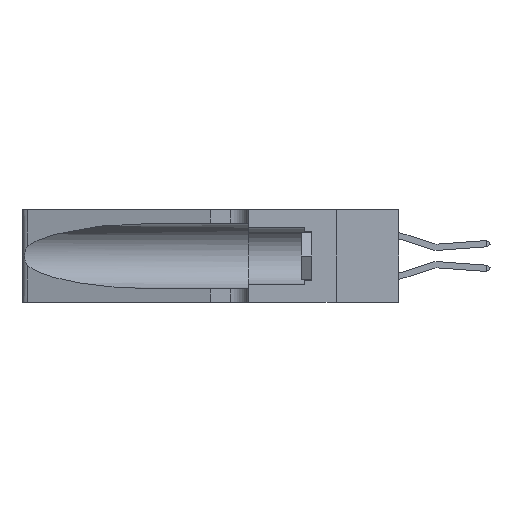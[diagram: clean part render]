
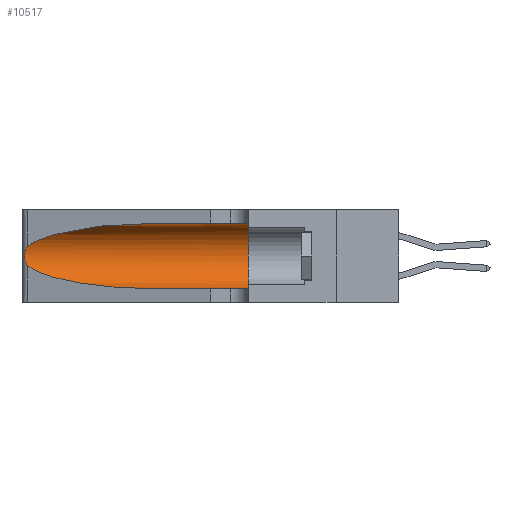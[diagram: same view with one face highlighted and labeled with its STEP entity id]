
A CAD part, left-side view. The second image highlights one B-rep face of the part: STEP entity #10517.
In plain terms, the highlighted cylindrical face has radius 3.308 mm (diameter 6.617 mm), a partial arc.
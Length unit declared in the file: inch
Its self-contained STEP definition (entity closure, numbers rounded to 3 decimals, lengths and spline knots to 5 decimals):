
#342 =( BOUNDED_CURVE ( )  B_SPLINE_CURVE ( 3, ( #559, #14095, #27897, #10256 ),
 .UNSPECIFIED., .F., .T. ) 
 B_SPLINE_CURVE_WITH_KNOTS ( ( 4, 4 ),
 ( 3.44316, 4.71239 ),
 .UNSPECIFIED. ) 
 CURVE ( )  GEOMETRIC_REPRESENTATION_ITEM ( )  RATIONAL_B_SPLINE_CURVE ( ( 1., 0.87, 0.87, 1. ) ) 
 REPRESENTATION_ITEM ( '' )  );
#559 = CARTESIAN_POINT ( 'NONE',  ( 0.25487, 1.22718, 0.14631 ) ) ;
#731 = CYLINDRICAL_SURFACE ( 'NONE', #2216, 0.13025 ) ;
#1449 =( BOUNDED_CURVE ( )  B_SPLINE_CURVE ( 3, ( #19832, #22501, #25131, #9156 ),
 .UNSPECIFIED., .F., .T. ) 
 B_SPLINE_CURVE_WITH_KNOTS ( ( 4, 4 ),
 ( 1.5708, 2.84003 ),
 .UNSPECIFIED. ) 
 CURVE ( )  GEOMETRIC_REPRESENTATION_ITEM ( )  RATIONAL_B_SPLINE_CURVE ( ( 1., 0.87, 0.87, 1. ) ) 
 REPRESENTATION_ITEM ( '' )  );
#1595 = DIRECTION ( 'NONE',  ( 0., 0., 1. ) ) ;
#1601 = FACE_OUTER_BOUND ( 'NONE', #4345, .T. ) ;
#1689 = EDGE_CURVE ( 'NONE', #8952, #18286, #342, .T. ) ;
#1985 = CARTESIAN_POINT ( 'NONE',  ( 0.26017, 1.23833, 0.17102 ) ) ;
#2048 = CARTESIAN_POINT ( 'NONE',  ( 0.1305, 0.72297, 0.31525 ) ) ;
#2216 = AXIS2_PLACEMENT_3D ( 'NONE', #30127, #14254, #8827 ) ;
#2761 = EDGE_CURVE ( 'NONE', #33352, #22773, #32976, .T. ) ;
#3137 = ORIENTED_EDGE ( 'NONE', *, *, #29196, .T. ) ;
#4345 = EDGE_LOOP ( 'NONE', ( #16651, #3137, #11198, #25383, #27033, #13718 ) ) ;
#4758 = CARTESIAN_POINT ( 'NONE',  ( 0.25789, 1.23486, 0.15765 ) ) ;
#5657 = VECTOR ( 'NONE', #19360, 39.37008 ) ;
#5799 = CARTESIAN_POINT ( 'NONE',  ( 0.1305, 1.61858, 0.31525 ) ) ;
#6446 = EDGE_CURVE ( 'NONE', #10162, #33352, #26591, .T. ) ;
#6543 = LINE ( 'NONE', #32476, #5657 ) ;
#6677 = CARTESIAN_POINT ( 'NONE',  ( 0.1305, 0.35, 0.05475 ) ) ;
#7495 = CARTESIAN_POINT ( 'NONE',  ( 0.25555, 1.22993, 0.14849 ) ) ;
#7801 = B_SPLINE_CURVE_WITH_KNOTS ( 'NONE', 3,
 ( #23412, #10077, #28714, #12760, #31333, #15485, #33938, #18200, #1985, #20864, #4758, #23508, #7495, #26157 ),
 .UNSPECIFIED., .F., .F.,
 ( 4, 2, 2, 2, 2, 2, 4 ),
 ( 0., 0.00027, 0.00053, 0.00107, 0.0016, 0.00187, 0.00214 ),
 .UNSPECIFIED. ) ;
#8508 = DIRECTION ( 'NONE',  ( 0., -1., 0. ) ) ;
#8827 = DIRECTION ( 'NONE',  ( 0., 0., -1. ) ) ;
#8952 = VERTEX_POINT ( 'NONE', #10320 ) ;
#9156 = CARTESIAN_POINT ( 'NONE',  ( 0.25487, 1.22718, 0.22369 ) ) ;
#10077 = CARTESIAN_POINT ( 'NONE',  ( 0.25555, 1.22994, 0.2215 ) ) ;
#10162 = VERTEX_POINT ( 'NONE', #2048 ) ;
#10256 = CARTESIAN_POINT ( 'NONE',  ( 0.1305, 0.72297, 0.05475 ) ) ;
#10320 = CARTESIAN_POINT ( 'NONE',  ( 0.25487, 1.22718, 0.14631 ) ) ;
#10517 = ADVANCED_FACE ( 'NONE', ( #1601 ), #731, .F. ) ;
#11198 = ORIENTED_EDGE ( 'NONE', *, *, #1689, .T. ) ;
#11284 = CARTESIAN_POINT ( 'NONE',  ( 0.1305, 0.72297, 0.05475 ) ) ;
#12760 = CARTESIAN_POINT ( 'NONE',  ( 0.25787, 1.23484, 0.2124 ) ) ;
#13718 = ORIENTED_EDGE ( 'NONE', *, *, #6446, .F. ) ;
#13776 = CARTESIAN_POINT ( 'NONE',  ( 0.1305, 0.35, 0.31525 ) ) ;
#14095 = CARTESIAN_POINT ( 'NONE',  ( 0.2373, 1.15595, 0.08982 ) ) ;
#14254 = DIRECTION ( 'NONE',  ( 0., -1., 0. ) ) ;
#15485 = CARTESIAN_POINT ( 'NONE',  ( 0.26018, 1.23835, 0.19895 ) ) ;
#16026 = VERTEX_POINT ( 'NONE', #32435 ) ;
#16651 = ORIENTED_EDGE ( 'NONE', *, *, #30262, .T. ) ;
#17809 = DIRECTION ( 'NONE',  ( 0., 1., 0. ) ) ;
#18200 = CARTESIAN_POINT ( 'NONE',  ( 0.26075, 1.23896, 0.178 ) ) ;
#18286 = VERTEX_POINT ( 'NONE', #11284 ) ;
#19360 = DIRECTION ( 'NONE',  ( 0., -1., 0. ) ) ;
#19583 = VECTOR ( 'NONE', #8508, 39.37008 ) ;
#19832 = CARTESIAN_POINT ( 'NONE',  ( 0.1305, 0.72297, 0.31525 ) ) ;
#20864 = CARTESIAN_POINT ( 'NONE',  ( 0.25856, 1.23593, 0.16098 ) ) ;
#22501 = CARTESIAN_POINT ( 'NONE',  ( 0.18966, 0.96281, 0.31525 ) ) ;
#22773 = VERTEX_POINT ( 'NONE', #6677 ) ;
#23412 = CARTESIAN_POINT ( 'NONE',  ( 0.25487, 1.22718, 0.22369 ) ) ;
#23508 = CARTESIAN_POINT ( 'NONE',  ( 0.25639, 1.23186, 0.15144 ) ) ;
#25131 = CARTESIAN_POINT ( 'NONE',  ( 0.2373, 1.15595, 0.28018 ) ) ;
#25383 = ORIENTED_EDGE ( 'NONE', *, *, #32046, .T. ) ;
#26157 = CARTESIAN_POINT ( 'NONE',  ( 0.25487, 1.22718, 0.14631 ) ) ;
#26591 = LINE ( 'NONE', #5799, #19583 ) ;
#27033 = ORIENTED_EDGE ( 'NONE', *, *, #2761, .F. ) ;
#27897 = CARTESIAN_POINT ( 'NONE',  ( 0.18966, 0.96281, 0.05475 ) ) ;
#28714 = CARTESIAN_POINT ( 'NONE',  ( 0.25639, 1.23184, 0.21858 ) ) ;
#29196 = EDGE_CURVE ( 'NONE', #16026, #8952, #7801, .T. ) ;
#30127 = CARTESIAN_POINT ( 'NONE',  ( 0.1305, 1.61858, 0.185 ) ) ;
#30262 = EDGE_CURVE ( 'NONE', #10162, #16026, #1449, .T. ) ;
#31333 = CARTESIAN_POINT ( 'NONE',  ( 0.25854, 1.2359, 0.20912 ) ) ;
#32046 = EDGE_CURVE ( 'NONE', #18286, #22773, #6543, .T. ) ;
#32435 = CARTESIAN_POINT ( 'NONE',  ( 0.25487, 1.22718, 0.22369 ) ) ;
#32476 = CARTESIAN_POINT ( 'NONE',  ( 0.1305, 1.61858, 0.05475 ) ) ;
#32976 = CIRCLE ( 'NONE', #33580, 0.13025 ) ;
#33352 = VERTEX_POINT ( 'NONE', #13776 ) ;
#33568 = CARTESIAN_POINT ( 'NONE',  ( 0.1305, 0.35, 0.185 ) ) ;
#33580 = AXIS2_PLACEMENT_3D ( 'NONE', #33568, #17809, #1595 ) ;
#33938 = CARTESIAN_POINT ( 'NONE',  ( 0.26075, 1.23896, 0.19203 ) ) ;
